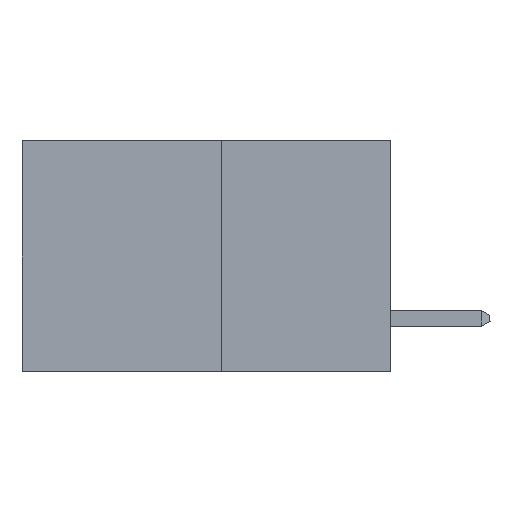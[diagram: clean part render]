
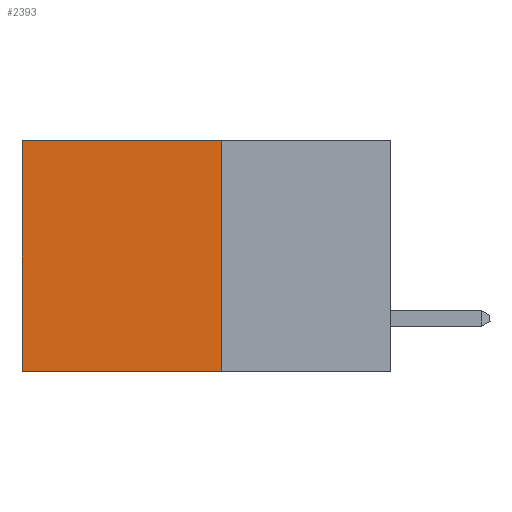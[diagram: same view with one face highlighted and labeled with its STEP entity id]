
A CAD part, left-side view. The second image highlights one B-rep face of the part: STEP entity #2393.
In plain terms, the highlighted planar face has unit normal (-1, 0, 0).
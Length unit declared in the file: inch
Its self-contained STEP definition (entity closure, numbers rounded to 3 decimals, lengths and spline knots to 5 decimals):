
#278 = ORIENTED_EDGE ( 'NONE', *, *, #25554, .F. ) ;
#433 = DIRECTION ( 'NONE',  ( 0., 0., -1. ) ) ;
#529 = CARTESIAN_POINT ( 'NONE',  ( 0.277, 0.27, -0.37 ) ) ;
#1940 = VECTOR ( 'NONE', #24289, 39.37008 ) ;
#2003 = EDGE_CURVE ( 'NONE', #3875, #27202, #22432, .T. ) ;
#2393 = ADVANCED_FACE ( 'NONE', ( #11086 ), #22285, .F. ) ;
#3351 = DIRECTION ( 'NONE',  ( 1., 0., 0. ) ) ;
#3397 = LINE ( 'NONE', #20117, #13890 ) ;
#3875 = VERTEX_POINT ( 'NONE', #12734 ) ;
#4097 = EDGE_CURVE ( 'NONE', #3875, #19597, #10145, .T. ) ;
#4800 = CARTESIAN_POINT ( 'NONE',  ( 0.277, 0.27, 0. ) ) ;
#5188 = ORIENTED_EDGE ( 'NONE', *, *, #2003, .T. ) ;
#6003 = CARTESIAN_POINT ( 'NONE',  ( 0.277, 0.59, 0. ) ) ;
#6628 = CARTESIAN_POINT ( 'NONE',  ( 0.277, 0.27, -0.37 ) ) ;
#6687 = DIRECTION ( 'NONE',  ( 0., 0., -1. ) ) ;
#6879 = LINE ( 'NONE', #9546, #1940 ) ;
#7307 = EDGE_CURVE ( 'NONE', #27202, #25793, #3397, .T. ) ;
#7949 = ORIENTED_EDGE ( 'NONE', *, *, #7307, .T. ) ;
#8430 = AXIS2_PLACEMENT_3D ( 'NONE', #6628, #3351, #6687 ) ;
#9546 = CARTESIAN_POINT ( 'NONE',  ( 0.277, 0.27, -0.37 ) ) ;
#9822 = VECTOR ( 'NONE', #19236, 39.37008 ) ;
#10145 = LINE ( 'NONE', #529, #26287 ) ;
#11086 = FACE_OUTER_BOUND ( 'NONE', #25248, .T. ) ;
#11557 = DIRECTION ( 'NONE',  ( 0., 0., -1. ) ) ;
#12734 = CARTESIAN_POINT ( 'NONE',  ( 0.277, 0.27, 0. ) ) ;
#13890 = VECTOR ( 'NONE', #11557, 39.37008 ) ;
#14293 = ORIENTED_EDGE ( 'NONE', *, *, #4097, .F. ) ;
#19236 = DIRECTION ( 'NONE',  ( 0., 1., 0. ) ) ;
#19597 = VERTEX_POINT ( 'NONE', #26257 ) ;
#20117 = CARTESIAN_POINT ( 'NONE',  ( 0.277, 0.59, -0.37 ) ) ;
#22285 = PLANE ( 'NONE',  #8430 ) ;
#22432 = LINE ( 'NONE', #4800, #9822 ) ;
#22858 = CARTESIAN_POINT ( 'NONE',  ( 0.277, 0.59, -0.37 ) ) ;
#24289 = DIRECTION ( 'NONE',  ( 0., 1., 0. ) ) ;
#25248 = EDGE_LOOP ( 'NONE', ( #7949, #278, #14293, #5188 ) ) ;
#25554 = EDGE_CURVE ( 'NONE', #19597, #25793, #6879, .T. ) ;
#25793 = VERTEX_POINT ( 'NONE', #22858 ) ;
#26257 = CARTESIAN_POINT ( 'NONE',  ( 0.277, 0.27, -0.37 ) ) ;
#26287 = VECTOR ( 'NONE', #433, 39.37008 ) ;
#27202 = VERTEX_POINT ( 'NONE', #6003 ) ;
